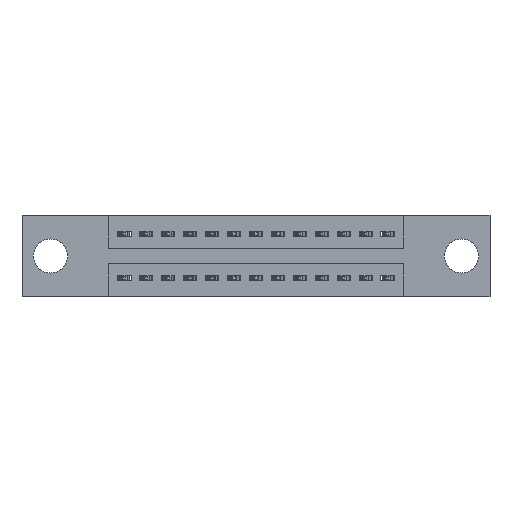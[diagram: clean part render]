
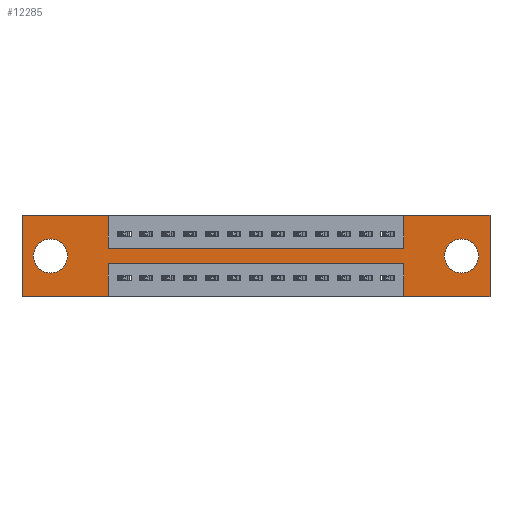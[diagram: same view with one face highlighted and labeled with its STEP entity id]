
A CAD part, front view. The second image highlights one B-rep face of the part: STEP entity #12285.
In plain terms, the highlighted planar face has unit normal (0, -1, 0).
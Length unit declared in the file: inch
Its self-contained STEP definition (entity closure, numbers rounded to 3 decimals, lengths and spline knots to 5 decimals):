
#157 = CARTESIAN_POINT ( 'NONE',  ( 0.13, 0., -0.185 ) ) ;
#213 = DIRECTION ( 'NONE',  ( 0., 0., 1. ) ) ;
#350 = DIRECTION ( 'NONE',  ( 0., 0., 1. ) ) ;
#573 = CARTESIAN_POINT ( 'NONE',  ( 0., 0., -0.37 ) ) ;
#646 = VERTEX_POINT ( 'NONE', #13337 ) ;
#663 = EDGE_LOOP ( 'NONE', ( #10200, #10763 ) ) ;
#757 = VERTEX_POINT ( 'NONE', #2731 ) ;
#815 = CIRCLE ( 'NONE', #1541, 0.078 ) ;
#1040 = VERTEX_POINT ( 'NONE', #2979 ) ;
#1123 = AXIS2_PLACEMENT_3D ( 'NONE', #8008, #5662, #13254 ) ;
#1153 = CARTESIAN_POINT ( 'NONE',  ( 0.13, 0., -0.263 ) ) ;
#1243 = VERTEX_POINT ( 'NONE', #12600 ) ;
#1342 = CARTESIAN_POINT ( 'NONE',  ( 2.005, 0., -0.107 ) ) ;
#1541 = AXIS2_PLACEMENT_3D ( 'NONE', #9302, #7156, #6159 ) ;
#1707 = VERTEX_POINT ( 'NONE', #1862 ) ;
#1862 = CARTESIAN_POINT ( 'NONE',  ( 1.7425, 0., 0. ) ) ;
#2085 = CARTESIAN_POINT ( 'NONE',  ( 0.3925, 0., -0.22 ) ) ;
#2086 = LINE ( 'NONE', #6460, #12277 ) ;
#2338 = EDGE_CURVE ( 'NONE', #1243, #13783, #4660, .T. ) ;
#2400 = CIRCLE ( 'NONE', #11887, 0.078 ) ;
#2403 = ORIENTED_EDGE ( 'NONE', *, *, #7842, .T. ) ;
#2462 = EDGE_CURVE ( 'NONE', #13783, #7065, #8454, .T. ) ;
#2612 = EDGE_CURVE ( 'NONE', #757, #5617, #5345, .T. ) ;
#2680 = DIRECTION ( 'NONE',  ( 0., 0., -1. ) ) ;
#2731 = CARTESIAN_POINT ( 'NONE',  ( 0., 0., 0. ) ) ;
#2814 = CIRCLE ( 'NONE', #1123, 0.078 ) ;
#2829 = CARTESIAN_POINT ( 'NONE',  ( 2.005, 0., -0.263 ) ) ;
#2979 = CARTESIAN_POINT ( 'NONE',  ( 0., 0., -0.37 ) ) ;
#3466 = LINE ( 'NONE', #12305, #7570 ) ;
#3491 = DIRECTION ( 'NONE',  ( 0., 1., 0. ) ) ;
#3733 = VERTEX_POINT ( 'NONE', #9748 ) ;
#3774 = LINE ( 'NONE', #9071, #7021 ) ;
#3852 = EDGE_CURVE ( 'NONE', #7341, #8329, #2400, .T. ) ;
#3868 = LINE ( 'NONE', #11114, #4206 ) ;
#4054 = EDGE_CURVE ( 'NONE', #13109, #1040, #3774, .T. ) ;
#4206 = VECTOR ( 'NONE', #6952, 39.37008 ) ;
#4233 = EDGE_LOOP ( 'NONE', ( #10802, #12517, #9335, #12495, #11025, #13515, #8532, #4974, #8897, #6070, #8549, #7225 ) ) ;
#4319 = FACE_OUTER_BOUND ( 'NONE', #4233, .T. ) ;
#4348 = VERTEX_POINT ( 'NONE', #6361 ) ;
#4456 = DIRECTION ( 'NONE',  ( 0., 0., -1. ) ) ;
#4477 = FACE_BOUND ( 'NONE', #12258, .T. ) ;
#4660 = LINE ( 'NONE', #6694, #10984 ) ;
#4974 = ORIENTED_EDGE ( 'NONE', *, *, #7224, .F. ) ;
#5113 = CARTESIAN_POINT ( 'NONE',  ( 0.13, 0., -0.107 ) ) ;
#5170 = VERTEX_POINT ( 'NONE', #5113 ) ;
#5177 = LINE ( 'NONE', #9763, #10653 ) ;
#5196 = VERTEX_POINT ( 'NONE', #1153 ) ;
#5345 = LINE ( 'NONE', #8727, #10477 ) ;
#5410 = CARTESIAN_POINT ( 'NONE',  ( 0., 0., 0. ) ) ;
#5520 = VECTOR ( 'NONE', #8417, 39.37008 ) ;
#5617 = VERTEX_POINT ( 'NONE', #9369 ) ;
#5621 = PLANE ( 'NONE',  #13713 ) ;
#5630 = DIRECTION ( 'NONE',  ( 0., 0., -1. ) ) ;
#5662 = DIRECTION ( 'NONE',  ( 0., 1., 0. ) ) ;
#5731 = LINE ( 'NONE', #7212, #9500 ) ;
#6017 = EDGE_CURVE ( 'NONE', #3733, #9905, #14128, .T. ) ;
#6070 = ORIENTED_EDGE ( 'NONE', *, *, #2612, .F. ) ;
#6159 = DIRECTION ( 'NONE',  ( 0., 0., -1. ) ) ;
#6361 = CARTESIAN_POINT ( 'NONE',  ( 1.7425, 0., -0.15 ) ) ;
#6460 = CARTESIAN_POINT ( 'NONE',  ( 0.3925, 0., 0. ) ) ;
#6477 = EDGE_CURVE ( 'NONE', #8329, #7341, #815, .T. ) ;
#6509 = DIRECTION ( 'NONE',  ( 1., 0., 0. ) ) ;
#6539 = DIRECTION ( 'NONE',  ( 1., 0., 0. ) ) ;
#6694 = CARTESIAN_POINT ( 'NONE',  ( 2.135, 0., 0. ) ) ;
#6782 = DIRECTION ( 'NONE',  ( -1., 0., 0. ) ) ;
#6952 = DIRECTION ( 'NONE',  ( 1., 0., 0. ) ) ;
#7021 = VECTOR ( 'NONE', #6782, 39.37008 ) ;
#7065 = VERTEX_POINT ( 'NONE', #8261 ) ;
#7156 = DIRECTION ( 'NONE',  ( 0., 1., 0. ) ) ;
#7212 = CARTESIAN_POINT ( 'NONE',  ( 1.7425, 0., 0. ) ) ;
#7224 = EDGE_CURVE ( 'NONE', #646, #4348, #3868, .T. ) ;
#7225 = ORIENTED_EDGE ( 'NONE', *, *, #4054, .F. ) ;
#7341 = VERTEX_POINT ( 'NONE', #2829 ) ;
#7570 = VECTOR ( 'NONE', #350, 39.37008 ) ;
#7782 = EDGE_CURVE ( 'NONE', #9905, #13109, #8976, .T. ) ;
#7842 = EDGE_CURVE ( 'NONE', #5170, #5196, #12003, .T. ) ;
#8008 = CARTESIAN_POINT ( 'NONE',  ( 0.13, 0., -0.185 ) ) ;
#8261 = CARTESIAN_POINT ( 'NONE',  ( 1.7425, 0., -0.37 ) ) ;
#8329 = VERTEX_POINT ( 'NONE', #1342 ) ;
#8417 = DIRECTION ( 'NONE',  ( -1., 0., 0. ) ) ;
#8454 = LINE ( 'NONE', #573, #5520 ) ;
#8474 = VECTOR ( 'NONE', #2680, 39.37008 ) ;
#8532 = ORIENTED_EDGE ( 'NONE', *, *, #11310, .F. ) ;
#8549 = ORIENTED_EDGE ( 'NONE', *, *, #9837, .F. ) ;
#8638 = CARTESIAN_POINT ( 'NONE',  ( 2.135, 0., -0.37 ) ) ;
#8727 = CARTESIAN_POINT ( 'NONE',  ( 0., 0., 0. ) ) ;
#8828 = CARTESIAN_POINT ( 'NONE',  ( 0., 0., -0.37 ) ) ;
#8897 = ORIENTED_EDGE ( 'NONE', *, *, #10529, .F. ) ;
#8976 = LINE ( 'NONE', #12419, #8474 ) ;
#9071 = CARTESIAN_POINT ( 'NONE',  ( 0., 0., -0.37 ) ) ;
#9302 = CARTESIAN_POINT ( 'NONE',  ( 2.005, 0., -0.185 ) ) ;
#9335 = ORIENTED_EDGE ( 'NONE', *, *, #13623, .F. ) ;
#9369 = CARTESIAN_POINT ( 'NONE',  ( 0.3925, 0., 0. ) ) ;
#9500 = VECTOR ( 'NONE', #9554, 39.37008 ) ;
#9514 = VECTOR ( 'NONE', #6509, 39.37008 ) ;
#9554 = DIRECTION ( 'NONE',  ( 0., 0., 1. ) ) ;
#9748 = CARTESIAN_POINT ( 'NONE',  ( 1.7425, 0., -0.22 ) ) ;
#9763 = CARTESIAN_POINT ( 'NONE',  ( 0., 0., 0. ) ) ;
#9837 = EDGE_CURVE ( 'NONE', #1040, #757, #5177, .T. ) ;
#9848 = LINE ( 'NONE', #5410, #9514 ) ;
#9850 = DIRECTION ( 'NONE',  ( 0., 1., 0. ) ) ;
#9890 = VECTOR ( 'NONE', #11237, 39.37008 ) ;
#9905 = VERTEX_POINT ( 'NONE', #2085 ) ;
#9946 = CARTESIAN_POINT ( 'NONE',  ( 2.005, 0., -0.185 ) ) ;
#10082 = CARTESIAN_POINT ( 'NONE',  ( 0.3925, 0., -0.22 ) ) ;
#10200 = ORIENTED_EDGE ( 'NONE', *, *, #6477, .T. ) ;
#10477 = VECTOR ( 'NONE', #6539, 39.37008 ) ;
#10529 = EDGE_CURVE ( 'NONE', #5617, #646, #2086, .T. ) ;
#10653 = VECTOR ( 'NONE', #13884, 39.37008 ) ;
#10763 = ORIENTED_EDGE ( 'NONE', *, *, #3852, .T. ) ;
#10802 = ORIENTED_EDGE ( 'NONE', *, *, #7782, .F. ) ;
#10923 = EDGE_CURVE ( 'NONE', #1707, #1243, #9848, .T. ) ;
#10984 = VECTOR ( 'NONE', #12040, 39.37008 ) ;
#11025 = ORIENTED_EDGE ( 'NONE', *, *, #2338, .F. ) ;
#11053 = DIRECTION ( 'NONE',  ( 0., -1., 0. ) ) ;
#11114 = CARTESIAN_POINT ( 'NONE',  ( 0.3925, 0., -0.15 ) ) ;
#11237 = DIRECTION ( 'NONE',  ( -1., 0., 0. ) ) ;
#11310 = EDGE_CURVE ( 'NONE', #4348, #1707, #5731, .T. ) ;
#11605 = EDGE_CURVE ( 'NONE', #5196, #5170, #2814, .T. ) ;
#11765 = DIRECTION ( 'NONE',  ( 0., 0., -1. ) ) ;
#11887 = AXIS2_PLACEMENT_3D ( 'NONE', #9946, #9850, #5630 ) ;
#12003 = CIRCLE ( 'NONE', #12196, 0.078 ) ;
#12040 = DIRECTION ( 'NONE',  ( 0., 0., -1. ) ) ;
#12196 = AXIS2_PLACEMENT_3D ( 'NONE', #157, #3491, #213 ) ;
#12258 = EDGE_LOOP ( 'NONE', ( #2403, #13814 ) ) ;
#12277 = VECTOR ( 'NONE', #11765, 39.37008 ) ;
#12285 = ADVANCED_FACE ( 'NONE', ( #12671, #4477, #4319 ), #5621, .T. ) ;
#12305 = CARTESIAN_POINT ( 'NONE',  ( 1.7425, 0., -0.37 ) ) ;
#12419 = CARTESIAN_POINT ( 'NONE',  ( 0.3925, 0., -0.37 ) ) ;
#12495 = ORIENTED_EDGE ( 'NONE', *, *, #2462, .F. ) ;
#12517 = ORIENTED_EDGE ( 'NONE', *, *, #6017, .F. ) ;
#12600 = CARTESIAN_POINT ( 'NONE',  ( 2.135, 0., 0. ) ) ;
#12671 = FACE_BOUND ( 'NONE', #663, .T. ) ;
#13109 = VERTEX_POINT ( 'NONE', #13195 ) ;
#13195 = CARTESIAN_POINT ( 'NONE',  ( 0.3925, 0., -0.37 ) ) ;
#13254 = DIRECTION ( 'NONE',  ( 0., 0., 1. ) ) ;
#13337 = CARTESIAN_POINT ( 'NONE',  ( 0.3925, 0., -0.15 ) ) ;
#13515 = ORIENTED_EDGE ( 'NONE', *, *, #10923, .F. ) ;
#13623 = EDGE_CURVE ( 'NONE', #7065, #3733, #3466, .T. ) ;
#13713 = AXIS2_PLACEMENT_3D ( 'NONE', #8828, #11053, #4456 ) ;
#13783 = VERTEX_POINT ( 'NONE', #8638 ) ;
#13814 = ORIENTED_EDGE ( 'NONE', *, *, #11605, .T. ) ;
#13884 = DIRECTION ( 'NONE',  ( 0., 0., 1. ) ) ;
#14128 = LINE ( 'NONE', #10082, #9890 ) ;
